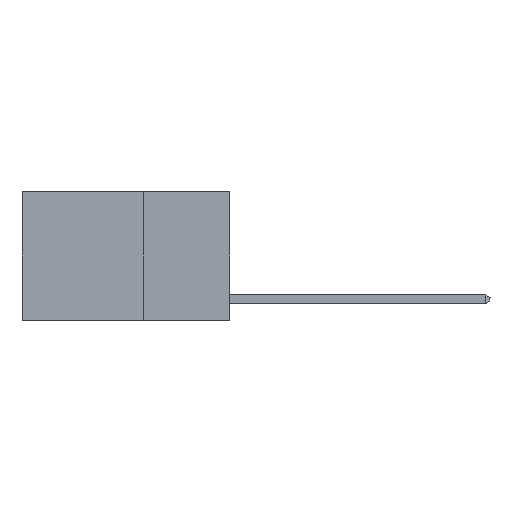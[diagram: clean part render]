
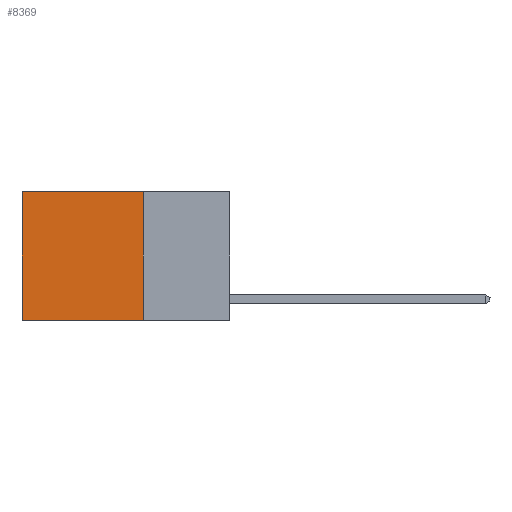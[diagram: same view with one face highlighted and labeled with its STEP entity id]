
A CAD part, left-side view. The second image highlights one B-rep face of the part: STEP entity #8369.
In plain terms, the highlighted planar face has unit normal (-1, 0, 0).
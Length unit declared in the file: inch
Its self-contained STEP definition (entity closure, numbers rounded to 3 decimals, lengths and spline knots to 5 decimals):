
#220 = FACE_OUTER_BOUND ( 'NONE', #22967, .T. ) ;
#757 = CARTESIAN_POINT ( 'NONE',  ( 0.2625, 0.25, -0.37 ) ) ;
#1298 = AXIS2_PLACEMENT_3D ( 'NONE', #6071, #1893, #13786 ) ;
#1893 = DIRECTION ( 'NONE',  ( 1., 0., 0. ) ) ;
#3046 = LINE ( 'NONE', #757, #8508 ) ;
#3056 = LINE ( 'NONE', #23956, #17261 ) ;
#3850 = ORIENTED_EDGE ( 'NONE', *, *, #16987, .T. ) ;
#6071 = CARTESIAN_POINT ( 'NONE',  ( 0.2625, 0.25, 0. ) ) ;
#7545 = EDGE_CURVE ( 'NONE', #24698, #24907, #3046, .T. ) ;
#8369 = ADVANCED_FACE ( 'NONE', ( #220 ), #11513, .F. ) ;
#8508 = VECTOR ( 'NONE', #14319, 39.37008 ) ;
#8716 = CARTESIAN_POINT ( 'NONE',  ( 0.2625, 0.6, 0. ) ) ;
#9240 = VERTEX_POINT ( 'NONE', #18023 ) ;
#10761 = DIRECTION ( 'NONE',  ( 0., 0., -1. ) ) ;
#11108 = VERTEX_POINT ( 'NONE', #8716 ) ;
#11173 = ORIENTED_EDGE ( 'NONE', *, *, #20179, .T. ) ;
#11513 = PLANE ( 'NONE',  #1298 ) ;
#11717 = EDGE_CURVE ( 'NONE', #9240, #24698, #16813, .T. ) ;
#13786 = DIRECTION ( 'NONE',  ( 0., 0., -1. ) ) ;
#14317 = ORIENTED_EDGE ( 'NONE', *, *, #7545, .F. ) ;
#14319 = DIRECTION ( 'NONE',  ( 0., 1., 0. ) ) ;
#14769 = DIRECTION ( 'NONE',  ( 0., 1., 0. ) ) ;
#16813 = LINE ( 'NONE', #24396, #23866 ) ;
#16987 = EDGE_CURVE ( 'NONE', #11108, #24907, #3056, .T. ) ;
#17063 = DIRECTION ( 'NONE',  ( 0., 0., -1. ) ) ;
#17261 = VECTOR ( 'NONE', #10761, 39.37008 ) ;
#18023 = CARTESIAN_POINT ( 'NONE',  ( 0.2625, 0.25, 0. ) ) ;
#18168 = CARTESIAN_POINT ( 'NONE',  ( 0.2625, 0.25, -0.37 ) ) ;
#19864 = LINE ( 'NONE', #22025, #23129 ) ;
#20104 = ORIENTED_EDGE ( 'NONE', *, *, #11717, .F. ) ;
#20179 = EDGE_CURVE ( 'NONE', #9240, #11108, #19864, .T. ) ;
#20669 = CARTESIAN_POINT ( 'NONE',  ( 0.2625, 0.6, -0.37 ) ) ;
#22025 = CARTESIAN_POINT ( 'NONE',  ( 0.2625, 0.25, 0. ) ) ;
#22967 = EDGE_LOOP ( 'NONE', ( #3850, #14317, #20104, #11173 ) ) ;
#23129 = VECTOR ( 'NONE', #14769, 39.37008 ) ;
#23866 = VECTOR ( 'NONE', #17063, 39.37008 ) ;
#23956 = CARTESIAN_POINT ( 'NONE',  ( 0.2625, 0.6, 0. ) ) ;
#24396 = CARTESIAN_POINT ( 'NONE',  ( 0.2625, 0.25, 0. ) ) ;
#24698 = VERTEX_POINT ( 'NONE', #18168 ) ;
#24907 = VERTEX_POINT ( 'NONE', #20669 ) ;
